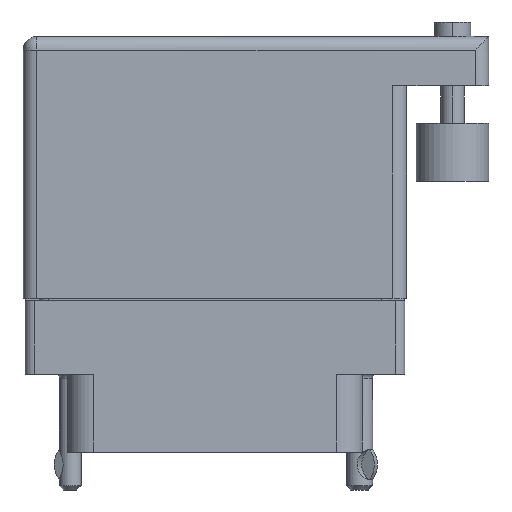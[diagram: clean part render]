
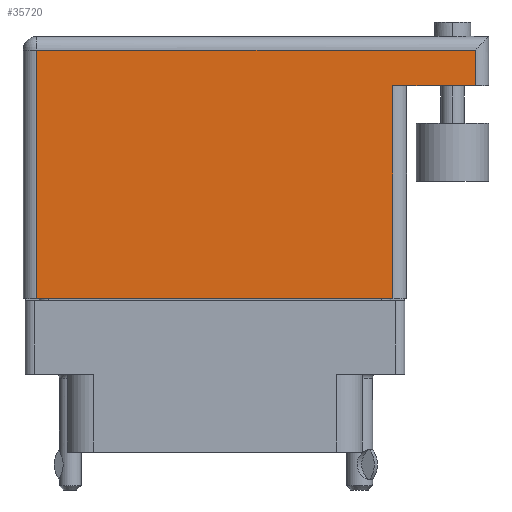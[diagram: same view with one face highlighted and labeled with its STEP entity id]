
A CAD part, front view. The second image highlights one B-rep face of the part: STEP entity #35720.
In plain terms, the highlighted face is planar.
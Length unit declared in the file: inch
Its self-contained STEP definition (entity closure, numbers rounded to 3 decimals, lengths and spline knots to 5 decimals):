
#793 = CARTESIAN_POINT ( 'NONE',  ( -0.6155, 0.759, 0.3575 ) ) ;
#902 = VERTEX_POINT ( 'NONE', #23630 ) ;
#1229 = LINE ( 'NONE', #14053, #33750 ) ;
#1833 = EDGE_CURVE ( 'NONE', #28805, #27137, #20233, .T. ) ;
#2177 = VERTEX_POINT ( 'NONE', #793 ) ;
#2747 = CARTESIAN_POINT ( 'NONE',  ( -0.6155, -0.1, 0.3575 ) ) ;
#2823 = DIRECTION ( 'NONE',  ( -1., 0., 0. ) ) ;
#3210 = EDGE_CURVE ( 'NONE', #902, #14153, #1229, .T. ) ;
#4671 = LINE ( 'NONE', #28192, #27498 ) ;
#7748 = CARTESIAN_POINT ( 'NONE',  ( 0.8995, 0.759, 0.3575 ) ) ;
#7843 = LINE ( 'NONE', #31058, #10295 ) ;
#7946 = EDGE_CURVE ( 'NONE', #26841, #2177, #4671, .T. ) ;
#7989 = LINE ( 'NONE', #2747, #40010 ) ;
#8357 = DIRECTION ( 'NONE',  ( 1., 0., 0. ) ) ;
#8946 = CARTESIAN_POINT ( 'NONE',  ( -0.6625, 0.806, 0.3575 ) ) ;
#10295 = VECTOR ( 'NONE', #38242, 39.37008 ) ;
#11966 = VECTOR ( 'NONE', #39342, 39.37008 ) ;
#12075 = CARTESIAN_POINT ( 'NONE',  ( 0.6155, 0.636, 0.3575 ) ) ;
#12138 = ORIENTED_EDGE ( 'NONE', *, *, #1833, .F. ) ;
#14053 = CARTESIAN_POINT ( 'NONE',  ( -0.6625, -0.1, 0.3575 ) ) ;
#14153 = VERTEX_POINT ( 'NONE', #38211 ) ;
#14571 = ORIENTED_EDGE ( 'NONE', *, *, #21452, .T. ) ;
#16248 = AXIS2_PLACEMENT_3D ( 'NONE', #8946, #30489, #2823 ) ;
#20233 = LINE ( 'NONE', #39612, #11966 ) ;
#21452 = EDGE_CURVE ( 'NONE', #2177, #902, #7989, .T. ) ;
#21467 = FACE_OUTER_BOUND ( 'NONE', #33127, .T. ) ;
#21591 = ORIENTED_EDGE ( 'NONE', *, *, #7946, .T. ) ;
#22418 = ORIENTED_EDGE ( 'NONE', *, *, #30502, .T. ) ;
#23630 = CARTESIAN_POINT ( 'NONE',  ( -0.6155, -0.1, 0.3575 ) ) ;
#26841 = VERTEX_POINT ( 'NONE', #7748 ) ;
#27137 = VERTEX_POINT ( 'NONE', #12075 ) ;
#27498 = VECTOR ( 'NONE', #31302, 39.37008 ) ;
#27584 = DIRECTION ( 'NONE',  ( 0., -1., 0. ) ) ;
#27801 = EDGE_CURVE ( 'NONE', #28805, #26841, #35229, .T. ) ;
#28190 = CARTESIAN_POINT ( 'NONE',  ( 0.8995, 0.806, 0.3575 ) ) ;
#28192 = CARTESIAN_POINT ( 'NONE',  ( -0.6625, 0.759, 0.3575 ) ) ;
#28805 = VERTEX_POINT ( 'NONE', #33553 ) ;
#29397 = VECTOR ( 'NONE', #34563, 39.37008 ) ;
#29784 = ORIENTED_EDGE ( 'NONE', *, *, #27801, .T. ) ;
#30489 = DIRECTION ( 'NONE',  ( 0., 0., -1. ) ) ;
#30502 = EDGE_CURVE ( 'NONE', #14153, #27137, #7843, .T. ) ;
#31058 = CARTESIAN_POINT ( 'NONE',  ( 0.6155, 0.636, 0.3575 ) ) ;
#31302 = DIRECTION ( 'NONE',  ( -1., 0., 0. ) ) ;
#32184 = ORIENTED_EDGE ( 'NONE', *, *, #3210, .T. ) ;
#33127 = EDGE_LOOP ( 'NONE', ( #32184, #22418, #12138, #29784, #21591, #14571 ) ) ;
#33553 = CARTESIAN_POINT ( 'NONE',  ( 0.8995, 0.636, 0.3575 ) ) ;
#33750 = VECTOR ( 'NONE', #8357, 39.37008 ) ;
#34563 = DIRECTION ( 'NONE',  ( 0., 1., 0. ) ) ;
#35229 = LINE ( 'NONE', #28190, #29397 ) ;
#35720 = ADVANCED_FACE ( 'NONE', ( #21467 ), #36883, .F. ) ;
#36883 = PLANE ( 'NONE',  #16248 ) ;
#38211 = CARTESIAN_POINT ( 'NONE',  ( 0.6155, -0.1, 0.3575 ) ) ;
#38242 = DIRECTION ( 'NONE',  ( 0., 1., 0. ) ) ;
#39342 = DIRECTION ( 'NONE',  ( -1., 0., 0. ) ) ;
#39612 = CARTESIAN_POINT ( 'NONE',  ( 0.9465, 0.636, 0.3575 ) ) ;
#40010 = VECTOR ( 'NONE', #27584, 39.37008 ) ;
